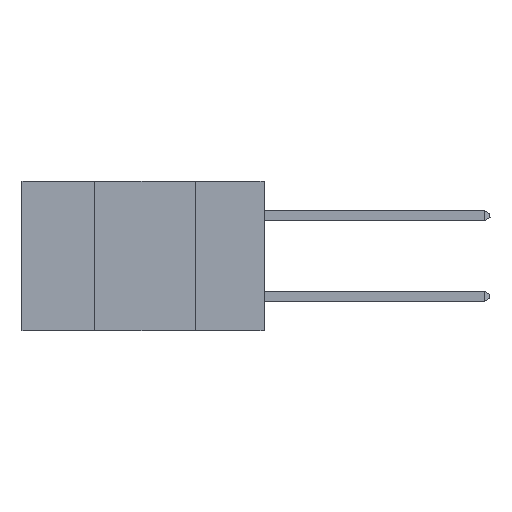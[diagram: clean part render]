
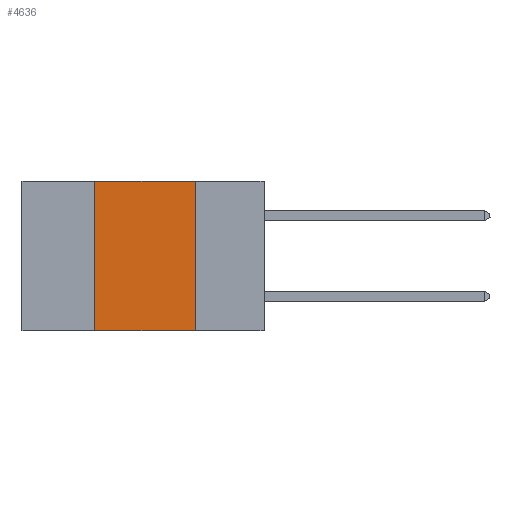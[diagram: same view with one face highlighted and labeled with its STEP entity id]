
A CAD part, left-side view. The second image highlights one B-rep face of the part: STEP entity #4636.
In plain terms, the highlighted planar face has unit normal (-1, 0, 0).
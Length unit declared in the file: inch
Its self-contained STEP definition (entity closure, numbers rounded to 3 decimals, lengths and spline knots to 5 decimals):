
#498 = CARTESIAN_POINT ( 'NONE',  ( 0., 0.6, 0. ) ) ;
#2062 = EDGE_CURVE ( 'NONE', #25493, #28808, #2202, .T. ) ;
#2202 = LINE ( 'NONE', #9774, #8185 ) ;
#2463 = ORIENTED_EDGE ( 'NONE', *, *, #23862, .T. ) ;
#2969 = CARTESIAN_POINT ( 'NONE',  ( 0., 0.42, -0.37 ) ) ;
#4150 = VERTEX_POINT ( 'NONE', #2969 ) ;
#4636 = ADVANCED_FACE ( 'NONE', ( #17825 ), #20011, .F. ) ;
#5202 = DIRECTION ( 'NONE',  ( 0., -1., 0. ) ) ;
#5293 = CARTESIAN_POINT ( 'NONE',  ( 0., 0.6, -0.37 ) ) ;
#5334 = EDGE_CURVE ( 'NONE', #28808, #8300, #21807, .T. ) ;
#5885 = CARTESIAN_POINT ( 'NONE',  ( 0., 0.42, 0. ) ) ;
#8185 = VECTOR ( 'NONE', #5202, 39.37008 ) ;
#8300 = VERTEX_POINT ( 'NONE', #25935 ) ;
#9023 = EDGE_LOOP ( 'NONE', ( #21242, #25325, #18911, #2463 ) ) ;
#9358 = DIRECTION ( 'NONE',  ( 0., 0., -1. ) ) ;
#9774 = CARTESIAN_POINT ( 'NONE',  ( 0., 0.6, 0. ) ) ;
#10530 = AXIS2_PLACEMENT_3D ( 'NONE', #498, #17554, #12567 ) ;
#12491 = CARTESIAN_POINT ( 'NONE',  ( 0., 0.42, 0. ) ) ;
#12567 = DIRECTION ( 'NONE',  ( 0., 0., -1. ) ) ;
#14627 = VECTOR ( 'NONE', #15123, 39.37008 ) ;
#15043 = CARTESIAN_POINT ( 'NONE',  ( 0., 0.17, 0. ) ) ;
#15123 = DIRECTION ( 'NONE',  ( 0., 0., 1. ) ) ;
#15859 = LINE ( 'NONE', #5293, #20033 ) ;
#16099 = EDGE_CURVE ( 'NONE', #4150, #25493, #17790, .T. ) ;
#16588 = VECTOR ( 'NONE', #9358, 39.37008 ) ;
#16790 = DIRECTION ( 'NONE',  ( 0., -1., 0. ) ) ;
#17554 = DIRECTION ( 'NONE',  ( 1., 0., 0. ) ) ;
#17790 = LINE ( 'NONE', #5885, #14627 ) ;
#17825 = FACE_OUTER_BOUND ( 'NONE', #9023, .T. ) ;
#18911 = ORIENTED_EDGE ( 'NONE', *, *, #16099, .F. ) ;
#20011 = PLANE ( 'NONE',  #10530 ) ;
#20033 = VECTOR ( 'NONE', #16790, 39.37008 ) ;
#20383 = CARTESIAN_POINT ( 'NONE',  ( 0., 0.17, 0. ) ) ;
#21242 = ORIENTED_EDGE ( 'NONE', *, *, #5334, .F. ) ;
#21807 = LINE ( 'NONE', #20383, #16588 ) ;
#23862 = EDGE_CURVE ( 'NONE', #4150, #8300, #15859, .T. ) ;
#25325 = ORIENTED_EDGE ( 'NONE', *, *, #2062, .F. ) ;
#25493 = VERTEX_POINT ( 'NONE', #12491 ) ;
#25935 = CARTESIAN_POINT ( 'NONE',  ( 0., 0.17, -0.37 ) ) ;
#28808 = VERTEX_POINT ( 'NONE', #15043 ) ;
